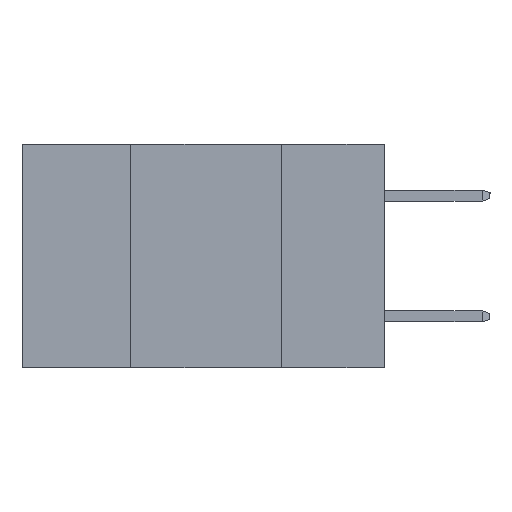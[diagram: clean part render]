
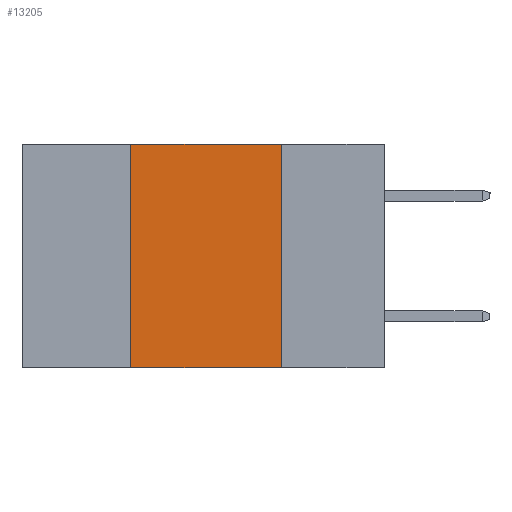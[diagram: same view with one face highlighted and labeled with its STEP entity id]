
A CAD part, left-side view. The second image highlights one B-rep face of the part: STEP entity #13205.
In plain terms, the highlighted planar face has unit normal (-1, 0, 0).
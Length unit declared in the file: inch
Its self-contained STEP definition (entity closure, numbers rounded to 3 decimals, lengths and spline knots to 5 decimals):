
#1926 = CARTESIAN_POINT ( 'NONE',  ( 0., 0.6, 0. ) ) ;
#1982 = VECTOR ( 'NONE', #20597, 39.37008 ) ;
#2091 = EDGE_CURVE ( 'NONE', #6604, #7581, #12669, .T. ) ;
#5172 = VERTEX_POINT ( 'NONE', #13934 ) ;
#5219 = PLANE ( 'NONE',  #16588 ) ;
#5637 = EDGE_CURVE ( 'NONE', #21099, #7581, #20919, .T. ) ;
#6025 = CARTESIAN_POINT ( 'NONE',  ( 0., 0.6, -0.37 ) ) ;
#6604 = VERTEX_POINT ( 'NONE', #18832 ) ;
#7082 = ORIENTED_EDGE ( 'NONE', *, *, #2091, .T. ) ;
#7509 = ORIENTED_EDGE ( 'NONE', *, *, #13983, .F. ) ;
#7581 = VERTEX_POINT ( 'NONE', #16262 ) ;
#7708 = DIRECTION ( 'NONE',  ( 0., -1., 0. ) ) ;
#8219 = DIRECTION ( 'NONE',  ( 0., 0., -1. ) ) ;
#8736 = DIRECTION ( 'NONE',  ( 0., -1., 0. ) ) ;
#9444 = VECTOR ( 'NONE', #14707, 39.37008 ) ;
#9642 = LINE ( 'NONE', #14376, #9444 ) ;
#10621 = ORIENTED_EDGE ( 'NONE', *, *, #12360, .F. ) ;
#10861 = ORIENTED_EDGE ( 'NONE', *, *, #5637, .F. ) ;
#11939 = FACE_OUTER_BOUND ( 'NONE', #16414, .T. ) ;
#12097 = CARTESIAN_POINT ( 'NONE',  ( 0., 0.17, -0.37 ) ) ;
#12360 = EDGE_CURVE ( 'NONE', #5172, #21099, #17284, .T. ) ;
#12669 = LINE ( 'NONE', #6025, #15551 ) ;
#13205 = ADVANCED_FACE ( 'NONE', ( #11939 ), #5219, .F. ) ;
#13934 = CARTESIAN_POINT ( 'NONE',  ( 0., 0.42, 0. ) ) ;
#13983 = EDGE_CURVE ( 'NONE', #6604, #5172, #9642, .T. ) ;
#14376 = CARTESIAN_POINT ( 'NONE',  ( 0., 0.42, -0.37 ) ) ;
#14707 = DIRECTION ( 'NONE',  ( 0., 0., 1. ) ) ;
#15198 = CARTESIAN_POINT ( 'NONE',  ( 0., 0.17, 0. ) ) ;
#15551 = VECTOR ( 'NONE', #7708, 39.37008 ) ;
#16262 = CARTESIAN_POINT ( 'NONE',  ( 0., 0.17, -0.37 ) ) ;
#16414 = EDGE_LOOP ( 'NONE', ( #10861, #10621, #7509, #7082 ) ) ;
#16588 = AXIS2_PLACEMENT_3D ( 'NONE', #21788, #18773, #8219 ) ;
#17284 = LINE ( 'NONE', #1926, #20341 ) ;
#18773 = DIRECTION ( 'NONE',  ( 1., 0., 0. ) ) ;
#18832 = CARTESIAN_POINT ( 'NONE',  ( 0., 0.42, -0.37 ) ) ;
#20341 = VECTOR ( 'NONE', #8736, 39.37008 ) ;
#20597 = DIRECTION ( 'NONE',  ( 0., 0., -1. ) ) ;
#20919 = LINE ( 'NONE', #12097, #1982 ) ;
#21099 = VERTEX_POINT ( 'NONE', #15198 ) ;
#21788 = CARTESIAN_POINT ( 'NONE',  ( 0., 0.6, 0. ) ) ;
